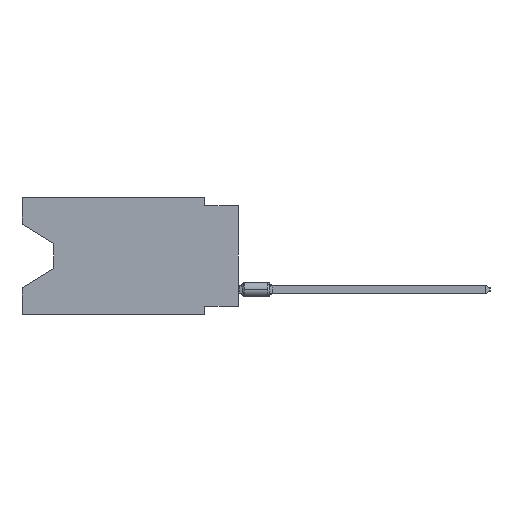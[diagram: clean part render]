
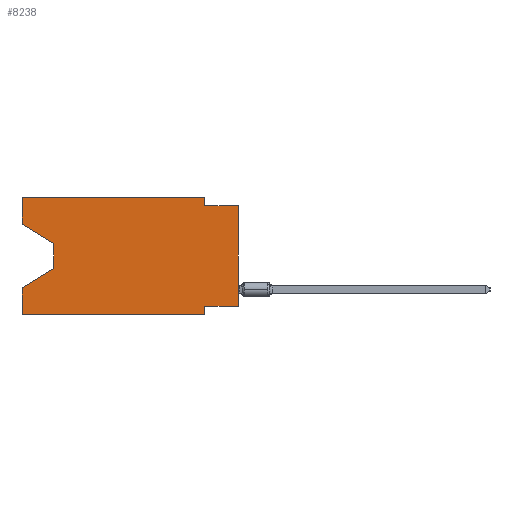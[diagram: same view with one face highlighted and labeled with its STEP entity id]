
A CAD part, left-side view. The second image highlights one B-rep face of the part: STEP entity #8238.
In plain terms, the highlighted planar face has unit normal (-1, 0, 0).
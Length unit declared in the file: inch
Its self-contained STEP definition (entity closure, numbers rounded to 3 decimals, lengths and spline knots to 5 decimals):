
#32 = DIRECTION ( 'NONE',  ( 1., 0., 0. ) ) ;
#49 = LINE ( 'NONE', #8975, #15796 ) ;
#63 = ORIENTED_EDGE ( 'NONE', *, *, #22048, .F. ) ;
#1391 = VERTEX_POINT ( 'NONE', #12443 ) ;
#1932 = CARTESIAN_POINT ( 'NONE',  ( 0., 0.645, -0.35 ) ) ;
#2535 = CARTESIAN_POINT ( 'NONE',  ( 0., 0.645, -0.08025 ) ) ;
#2995 = ORIENTED_EDGE ( 'NONE', *, *, #6276, .T. ) ;
#3144 = VERTEX_POINT ( 'NONE', #28324 ) ;
#3393 = CARTESIAN_POINT ( 'NONE',  ( 0., 0.645, -0.26975 ) ) ;
#3407 = ORIENTED_EDGE ( 'NONE', *, *, #18899, .T. ) ;
#3966 = EDGE_CURVE ( 'NONE', #17884, #1391, #14612, .T. ) ;
#4495 = DIRECTION ( 'NONE',  ( 0., -1., 0. ) ) ;
#5131 = VERTEX_POINT ( 'NONE', #27191 ) ;
#5348 = ORIENTED_EDGE ( 'NONE', *, *, #26700, .T. ) ;
#5547 = EDGE_CURVE ( 'NONE', #20322, #6521, #22321, .T. ) ;
#6276 = EDGE_CURVE ( 'NONE', #15649, #5131, #8591, .T. ) ;
#6521 = VERTEX_POINT ( 'NONE', #13094 ) ;
#6619 = EDGE_CURVE ( 'NONE', #10885, #17185, #9424, .T. ) ;
#6767 = DIRECTION ( 'NONE',  ( 0., 0., -1. ) ) ;
#6857 = VECTOR ( 'NONE', #18355, 39.37008 ) ;
#6943 = CARTESIAN_POINT ( 'NONE',  ( 0., 0.1, 0. ) ) ;
#7674 = VECTOR ( 'NONE', #23364, 39.37008 ) ;
#8238 = ADVANCED_FACE ( 'NONE', ( #26822 ), #17891, .F. ) ;
#8591 = LINE ( 'NONE', #28965, #16428 ) ;
#8975 = CARTESIAN_POINT ( 'NONE',  ( 0., 0.645, 0. ) ) ;
#9100 = EDGE_CURVE ( 'NONE', #5131, #15034, #17194, .T. ) ;
#9424 = LINE ( 'NONE', #6943, #23434 ) ;
#9638 = LINE ( 'NONE', #27529, #24672 ) ;
#9680 = CARTESIAN_POINT ( 'NONE',  ( 0., 0.645, -0.35 ) ) ;
#10077 = ORIENTED_EDGE ( 'NONE', *, *, #13535, .F. ) ;
#10089 = DIRECTION ( 'NONE',  ( 0., 0., 1. ) ) ;
#10174 = ORIENTED_EDGE ( 'NONE', *, *, #9100, .T. ) ;
#10711 = CARTESIAN_POINT ( 'NONE',  ( 0., 0., -0.325 ) ) ;
#10885 = VERTEX_POINT ( 'NONE', #23491 ) ;
#11137 = EDGE_CURVE ( 'NONE', #20322, #15034, #49, .T. ) ;
#11158 = CARTESIAN_POINT ( 'NONE',  ( 0., 0.645, 0. ) ) ;
#11896 = LINE ( 'NONE', #12048, #22924 ) ;
#12024 = LINE ( 'NONE', #14219, #14337 ) ;
#12048 = CARTESIAN_POINT ( 'NONE',  ( 0., 0.645, 0. ) ) ;
#12415 = DIRECTION ( 'NONE',  ( 0., 0., 1. ) ) ;
#12443 = CARTESIAN_POINT ( 'NONE',  ( 0., 0.645, 0. ) ) ;
#13094 = CARTESIAN_POINT ( 'NONE',  ( 0., 0.1, -0.35 ) ) ;
#13107 = ORIENTED_EDGE ( 'NONE', *, *, #3966, .F. ) ;
#13535 = EDGE_CURVE ( 'NONE', #1391, #10885, #11896, .T. ) ;
#14219 = CARTESIAN_POINT ( 'NONE',  ( 0., 0., 0. ) ) ;
#14337 = VECTOR ( 'NONE', #10089, 39.37008 ) ;
#14555 = VECTOR ( 'NONE', #16291, 39.37008 ) ;
#14612 = LINE ( 'NONE', #21641, #24737 ) ;
#14807 = ORIENTED_EDGE ( 'NONE', *, *, #11137, .F. ) ;
#15034 = VERTEX_POINT ( 'NONE', #3393 ) ;
#15649 = VERTEX_POINT ( 'NONE', #24831 ) ;
#15796 = VECTOR ( 'NONE', #17908, 39.37008 ) ;
#16150 = DIRECTION ( 'NONE',  ( 0., -1., 0. ) ) ;
#16291 = DIRECTION ( 'NONE',  ( 0., -1., 0. ) ) ;
#16322 = ORIENTED_EDGE ( 'NONE', *, *, #25000, .F. ) ;
#16428 = VECTOR ( 'NONE', #24418, 39.37008 ) ;
#17185 = VERTEX_POINT ( 'NONE', #27282 ) ;
#17192 = VECTOR ( 'NONE', #4495, 39.37008 ) ;
#17194 = LINE ( 'NONE', #18942, #7674 ) ;
#17884 = VERTEX_POINT ( 'NONE', #25415 ) ;
#17891 = PLANE ( 'NONE',  #22637 ) ;
#17908 = DIRECTION ( 'NONE',  ( 0., 0., 1. ) ) ;
#18355 = DIRECTION ( 'NONE',  ( 0., -0.855, -0.519 ) ) ;
#18489 = VERTEX_POINT ( 'NONE', #18792 ) ;
#18689 = VERTEX_POINT ( 'NONE', #10711 ) ;
#18792 = CARTESIAN_POINT ( 'NONE',  ( 0., 0., -0.025 ) ) ;
#18810 = ORIENTED_EDGE ( 'NONE', *, *, #5547, .T. ) ;
#18899 = EDGE_CURVE ( 'NONE', #18689, #18489, #12024, .T. ) ;
#18942 = CARTESIAN_POINT ( 'NONE',  ( 0., 0.55, -0.212 ) ) ;
#19019 = EDGE_LOOP ( 'NONE', ( #5348, #2995, #10174, #14807, #18810, #63, #16322, #3407, #25943, #22094, #10077, #13107 ) ) ;
#20322 = VERTEX_POINT ( 'NONE', #1932 ) ;
#21641 = CARTESIAN_POINT ( 'NONE',  ( 0., 0.645, 0. ) ) ;
#22048 = EDGE_CURVE ( 'NONE', #3144, #6521, #9638, .T. ) ;
#22094 = ORIENTED_EDGE ( 'NONE', *, *, #6619, .F. ) ;
#22321 = LINE ( 'NONE', #9680, #14555 ) ;
#22332 = CARTESIAN_POINT ( 'NONE',  ( 0., 0., -0.325 ) ) ;
#22637 = AXIS2_PLACEMENT_3D ( 'NONE', #11158, #32, #6767 ) ;
#22924 = VECTOR ( 'NONE', #16150, 39.37008 ) ;
#23158 = VECTOR ( 'NONE', #24076, 39.37008 ) ;
#23364 = DIRECTION ( 'NONE',  ( 0., 0.855, -0.519 ) ) ;
#23434 = VECTOR ( 'NONE', #26996, 39.37008 ) ;
#23491 = CARTESIAN_POINT ( 'NONE',  ( 0., 0.1, 0. ) ) ;
#24076 = DIRECTION ( 'NONE',  ( 0., 1., 0. ) ) ;
#24247 = LINE ( 'NONE', #22332, #23158 ) ;
#24418 = DIRECTION ( 'NONE',  ( 0., 0., -1. ) ) ;
#24672 = VECTOR ( 'NONE', #27802, 39.37008 ) ;
#24737 = VECTOR ( 'NONE', #12415, 39.37008 ) ;
#24801 = LINE ( 'NONE', #2535, #6857 ) ;
#24831 = CARTESIAN_POINT ( 'NONE',  ( 0., 0.55, -0.138 ) ) ;
#25000 = EDGE_CURVE ( 'NONE', #18689, #3144, #24247, .T. ) ;
#25415 = CARTESIAN_POINT ( 'NONE',  ( 0., 0.645, -0.08025 ) ) ;
#25943 = ORIENTED_EDGE ( 'NONE', *, *, #28657, .F. ) ;
#26327 = LINE ( 'NONE', #26466, #17192 ) ;
#26466 = CARTESIAN_POINT ( 'NONE',  ( 0., 0., -0.025 ) ) ;
#26700 = EDGE_CURVE ( 'NONE', #17884, #15649, #24801, .T. ) ;
#26822 = FACE_OUTER_BOUND ( 'NONE', #19019, .T. ) ;
#26996 = DIRECTION ( 'NONE',  ( 0., 0., -1. ) ) ;
#27191 = CARTESIAN_POINT ( 'NONE',  ( 0., 0.55, -0.212 ) ) ;
#27282 = CARTESIAN_POINT ( 'NONE',  ( 0., 0.1, -0.025 ) ) ;
#27529 = CARTESIAN_POINT ( 'NONE',  ( 0., 0.1, -0.35 ) ) ;
#27802 = DIRECTION ( 'NONE',  ( 0., 0., -1. ) ) ;
#28324 = CARTESIAN_POINT ( 'NONE',  ( 0., 0.1, -0.325 ) ) ;
#28657 = EDGE_CURVE ( 'NONE', #17185, #18489, #26327, .T. ) ;
#28965 = CARTESIAN_POINT ( 'NONE',  ( 0., 0.55, -0.138 ) ) ;
